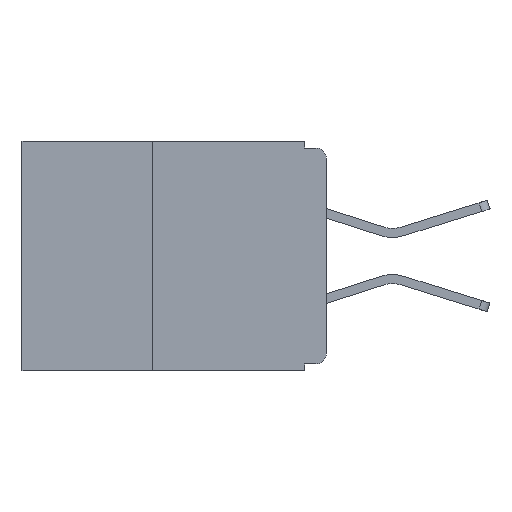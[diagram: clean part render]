
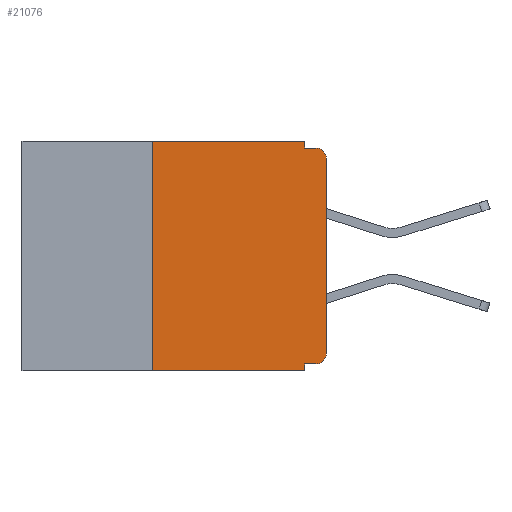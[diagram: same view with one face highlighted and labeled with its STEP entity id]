
A CAD part, left-side view. The second image highlights one B-rep face of the part: STEP entity #21076.
In plain terms, the highlighted planar face has unit normal (-1, 0, 0).
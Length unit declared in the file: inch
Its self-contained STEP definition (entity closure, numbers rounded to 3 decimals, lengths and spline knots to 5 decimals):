
#216 = LINE ( 'NONE', #3592, #23913 ) ;
#339 = DIRECTION ( 'NONE',  ( 0., 0., -1. ) ) ;
#919 = VERTEX_POINT ( 'NONE', #5137 ) ;
#1031 = DIRECTION ( 'NONE',  ( 0., -1., 0. ) ) ;
#1328 = EDGE_LOOP ( 'NONE', ( #28566, #8560, #25838, #28643, #7196, #28317, #28672, #26664, #5871, #19528 ) ) ;
#1437 = CARTESIAN_POINT ( 'NONE',  ( 0., 0.437, 0. ) ) ;
#2125 = VECTOR ( 'NONE', #8510, 39.37008 ) ;
#2825 = CARTESIAN_POINT ( 'NONE',  ( 0., 0.015, -0.01 ) ) ;
#3340 = AXIS2_PLACEMENT_3D ( 'NONE', #24168, #10423, #26441 ) ;
#3409 = CARTESIAN_POINT ( 'NONE',  ( 0., 0.031, 0. ) ) ;
#3450 = VERTEX_POINT ( 'NONE', #2825 ) ;
#3592 = CARTESIAN_POINT ( 'NONE',  ( 0., 0.437, 0. ) ) ;
#3636 = VERTEX_POINT ( 'NONE', #28663 ) ;
#3709 = PLANE ( 'NONE',  #12609 ) ;
#3906 = CARTESIAN_POINT ( 'NONE',  ( 0., 0., -0.01 ) ) ;
#4066 = LINE ( 'NONE', #7943, #21677 ) ;
#4268 = EDGE_CURVE ( 'NONE', #23024, #25870, #4066, .T. ) ;
#5115 = DIRECTION ( 'NONE',  ( 0., 1., 0. ) ) ;
#5137 = CARTESIAN_POINT ( 'NONE',  ( 0., 0.015, -0.32 ) ) ;
#5472 = VECTOR ( 'NONE', #5115, 39.37008 ) ;
#5871 = ORIENTED_EDGE ( 'NONE', *, *, #18685, .F. ) ;
#6165 = VERTEX_POINT ( 'NONE', #27272 ) ;
#6447 = CARTESIAN_POINT ( 'NONE',  ( 0., 0.031, -0.33 ) ) ;
#6765 = CARTESIAN_POINT ( 'NONE',  ( 0., 0.031, -0.33 ) ) ;
#7196 = ORIENTED_EDGE ( 'NONE', *, *, #8846, .F. ) ;
#7539 = LINE ( 'NONE', #3906, #25214 ) ;
#7672 = CARTESIAN_POINT ( 'NONE',  ( 0., 0.437, -0.33 ) ) ;
#7943 = CARTESIAN_POINT ( 'NONE',  ( 0., 0., 0. ) ) ;
#8292 = DIRECTION ( 'NONE',  ( 1., 0., 0. ) ) ;
#8419 = CIRCLE ( 'NONE', #3340, 0.015 ) ;
#8510 = DIRECTION ( 'NONE',  ( 0., 0., 1. ) ) ;
#8560 = ORIENTED_EDGE ( 'NONE', *, *, #14115, .T. ) ;
#8846 = EDGE_CURVE ( 'NONE', #6165, #10891, #216, .T. ) ;
#8895 = VECTOR ( 'NONE', #1031, 39.37008 ) ;
#9085 = DIRECTION ( 'NONE',  ( 0., 0., -1. ) ) ;
#9291 = CIRCLE ( 'NONE', #27052, 0.015 ) ;
#9458 = EDGE_CURVE ( 'NONE', #919, #23024, #8419, .T. ) ;
#10334 = DIRECTION ( 'NONE',  ( 0., 0., 1. ) ) ;
#10423 = DIRECTION ( 'NONE',  ( -1., 0., 0. ) ) ;
#10891 = VERTEX_POINT ( 'NONE', #11072 ) ;
#11072 = CARTESIAN_POINT ( 'NONE',  ( 0., 0.031, 0. ) ) ;
#11615 = LINE ( 'NONE', #23392, #5472 ) ;
#12609 = AXIS2_PLACEMENT_3D ( 'NONE', #1437, #8292, #24433 ) ;
#12759 = EDGE_CURVE ( 'NONE', #3636, #13323, #19458, .T. ) ;
#12966 = FACE_OUTER_BOUND ( 'NONE', #1328, .T. ) ;
#13323 = VERTEX_POINT ( 'NONE', #6447 ) ;
#14081 = DIRECTION ( 'NONE',  ( -1., 0., 0. ) ) ;
#14115 = EDGE_CURVE ( 'NONE', #25870, #3450, #9291, .T. ) ;
#14180 = CARTESIAN_POINT ( 'NONE',  ( 0., 0.031, -0.01 ) ) ;
#14297 = EDGE_CURVE ( 'NONE', #21530, #13323, #21150, .T. ) ;
#14338 = LINE ( 'NONE', #24642, #2125 ) ;
#15282 = DIRECTION ( 'NONE',  ( 0., -1., 0. ) ) ;
#15829 = EDGE_CURVE ( 'NONE', #21530, #6165, #14338, .T. ) ;
#16019 = CARTESIAN_POINT ( 'NONE',  ( 0., 0., -0.305 ) ) ;
#16069 = VERTEX_POINT ( 'NONE', #14180 ) ;
#17327 = VECTOR ( 'NONE', #9085, 39.37008 ) ;
#18058 = VECTOR ( 'NONE', #28573, 39.37008 ) ;
#18090 = CARTESIAN_POINT ( 'NONE',  ( 0., 0., -0.025 ) ) ;
#18685 = EDGE_CURVE ( 'NONE', #919, #3636, #11615, .T. ) ;
#18864 = EDGE_CURVE ( 'NONE', #10891, #16069, #24184, .T. ) ;
#19458 = LINE ( 'NONE', #6765, #17327 ) ;
#19528 = ORIENTED_EDGE ( 'NONE', *, *, #9458, .T. ) ;
#21076 = ADVANCED_FACE ( 'NONE', ( #12966 ), #3709, .F. ) ;
#21150 = LINE ( 'NONE', #7672, #8895 ) ;
#21466 = CARTESIAN_POINT ( 'NONE',  ( 0., 0.25, -0.33 ) ) ;
#21530 = VERTEX_POINT ( 'NONE', #21466 ) ;
#21677 = VECTOR ( 'NONE', #10334, 39.37008 ) ;
#23024 = VERTEX_POINT ( 'NONE', #16019 ) ;
#23392 = CARTESIAN_POINT ( 'NONE',  ( 0., 0., -0.32 ) ) ;
#23913 = VECTOR ( 'NONE', #24316, 39.37008 ) ;
#24168 = CARTESIAN_POINT ( 'NONE',  ( 0., 0.015, -0.305 ) ) ;
#24184 = LINE ( 'NONE', #3409, #18058 ) ;
#24316 = DIRECTION ( 'NONE',  ( 0., -1., 0. ) ) ;
#24433 = DIRECTION ( 'NONE',  ( 0., 0., -1. ) ) ;
#24642 = CARTESIAN_POINT ( 'NONE',  ( 0., 0.25, -0.33 ) ) ;
#25214 = VECTOR ( 'NONE', #15282, 39.37008 ) ;
#25838 = ORIENTED_EDGE ( 'NONE', *, *, #26395, .F. ) ;
#25870 = VERTEX_POINT ( 'NONE', #18090 ) ;
#26395 = EDGE_CURVE ( 'NONE', #16069, #3450, #7539, .T. ) ;
#26441 = DIRECTION ( 'NONE',  ( 0., 0., -1. ) ) ;
#26664 = ORIENTED_EDGE ( 'NONE', *, *, #12759, .F. ) ;
#27052 = AXIS2_PLACEMENT_3D ( 'NONE', #27733, #14081, #339 ) ;
#27272 = CARTESIAN_POINT ( 'NONE',  ( 0., 0.25, 0. ) ) ;
#27733 = CARTESIAN_POINT ( 'NONE',  ( 0., 0.015, -0.025 ) ) ;
#28317 = ORIENTED_EDGE ( 'NONE', *, *, #15829, .F. ) ;
#28566 = ORIENTED_EDGE ( 'NONE', *, *, #4268, .T. ) ;
#28573 = DIRECTION ( 'NONE',  ( 0., 0., -1. ) ) ;
#28643 = ORIENTED_EDGE ( 'NONE', *, *, #18864, .F. ) ;
#28663 = CARTESIAN_POINT ( 'NONE',  ( 0., 0.031, -0.32 ) ) ;
#28672 = ORIENTED_EDGE ( 'NONE', *, *, #14297, .T. ) ;
